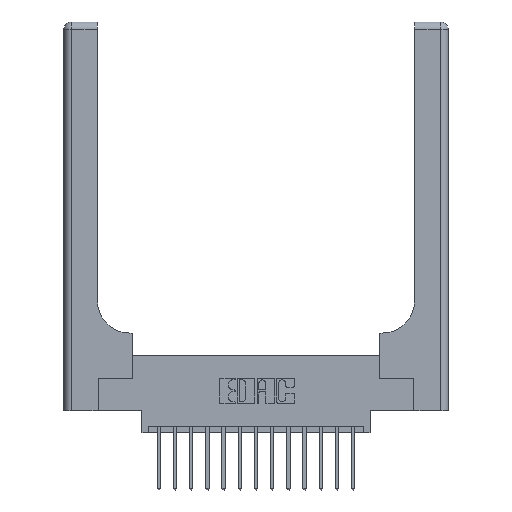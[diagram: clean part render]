
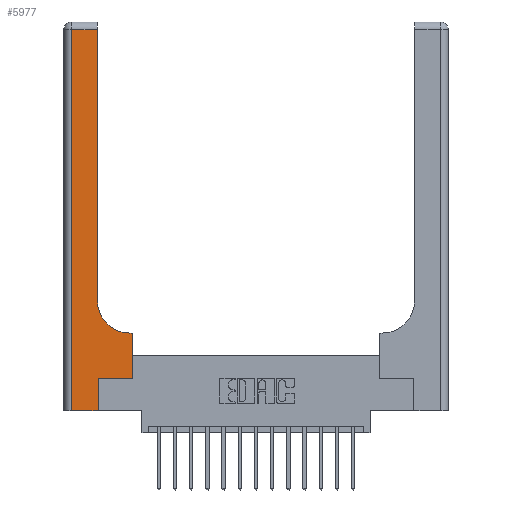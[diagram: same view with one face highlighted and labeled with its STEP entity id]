
A CAD part, top view. The second image highlights one B-rep face of the part: STEP entity #5977.
In plain terms, the highlighted planar face has unit normal (0, 0, 1).
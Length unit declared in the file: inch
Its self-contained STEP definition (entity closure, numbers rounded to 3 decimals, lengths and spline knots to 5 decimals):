
#105 = EDGE_CURVE ( 'NONE', #8761, #6554, #12553, .T. ) ;
#276 = EDGE_CURVE ( 'NONE', #6554, #7786, #18009, .T. ) ;
#674 = CARTESIAN_POINT ( 'NONE',  ( 0.06, 0., 0.37 ) ) ;
#1154 = ORIENTED_EDGE ( 'NONE', *, *, #7341, .T. ) ;
#1285 = EDGE_CURVE ( 'NONE', #2473, #6010, #10579, .T. ) ;
#1869 = AXIS2_PLACEMENT_3D ( 'NONE', #15434, #2851, #9680 ) ;
#2473 = VERTEX_POINT ( 'NONE', #8098 ) ;
#2480 = CARTESIAN_POINT ( 'NONE',  ( 0.26, 0.85, 0.37 ) ) ;
#2680 = DIRECTION ( 'NONE',  ( 0., 1., 0. ) ) ;
#2851 = DIRECTION ( 'NONE',  ( 0., 0., -1. ) ) ;
#3140 = DIRECTION ( 'NONE',  ( -1., 0., 0. ) ) ;
#3757 = VECTOR ( 'NONE', #4029, 39.37008 ) ;
#3887 = CARTESIAN_POINT ( 'NONE',  ( 0.265, 0., 0.37 ) ) ;
#3974 = LINE ( 'NONE', #3887, #14321 ) ;
#4029 = DIRECTION ( 'NONE',  ( 1., 0., 0. ) ) ;
#4353 = CARTESIAN_POINT ( 'NONE',  ( 0.26, 2.94, 0.37 ) ) ;
#4377 = LINE ( 'NONE', #7072, #3757 ) ;
#4520 = FACE_OUTER_BOUND ( 'NONE', #8047, .T. ) ;
#4982 = VECTOR ( 'NONE', #13230, 39.37008 ) ;
#5689 = EDGE_CURVE ( 'NONE', #13192, #17780, #13564, .T. ) ;
#5850 = CARTESIAN_POINT ( 'NONE',  ( 0.51, 0.6, 0.37 ) ) ;
#5942 = EDGE_CURVE ( 'NONE', #17780, #8761, #7209, .T. ) ;
#5977 = ADVANCED_FACE ( 'NONE', ( #4520 ), #10151, .F. ) ;
#6010 = VERTEX_POINT ( 'NONE', #674 ) ;
#6452 = CARTESIAN_POINT ( 'NONE',  ( 0.265, 0.25, 0.37 ) ) ;
#6554 = VERTEX_POINT ( 'NONE', #5850 ) ;
#7072 = CARTESIAN_POINT ( 'NONE',  ( 0., 0., 0.37 ) ) ;
#7209 = LINE ( 'NONE', #15556, #10176 ) ;
#7341 = EDGE_CURVE ( 'NONE', #9785, #13192, #3974, .T. ) ;
#7627 = CARTESIAN_POINT ( 'NONE',  ( 0., 2.94, 0.37 ) ) ;
#7652 = VECTOR ( 'NONE', #15150, 39.37008 ) ;
#7786 = VERTEX_POINT ( 'NONE', #2480 ) ;
#7792 = ORIENTED_EDGE ( 'NONE', *, *, #105, .T. ) ;
#7852 = EDGE_CURVE ( 'NONE', #7786, #9629, #8100, .T. ) ;
#7862 = DIRECTION ( 'NONE',  ( 1., 0., 0. ) ) ;
#7957 = CARTESIAN_POINT ( 'NONE',  ( 0.265, 0.25, 0.37 ) ) ;
#8010 = ORIENTED_EDGE ( 'NONE', *, *, #5942, .T. ) ;
#8047 = EDGE_LOOP ( 'NONE', ( #18118, #9099, #8105, #12429, #1154, #12051, #8010, #7792, #12926 ) ) ;
#8098 = CARTESIAN_POINT ( 'NONE',  ( 0.06, 2.94, 0.37 ) ) ;
#8100 = LINE ( 'NONE', #11119, #7652 ) ;
#8105 = ORIENTED_EDGE ( 'NONE', *, *, #1285, .T. ) ;
#8761 = VERTEX_POINT ( 'NONE', #17090 ) ;
#9042 = AXIS2_PLACEMENT_3D ( 'NONE', #15741, #15841, #3140 ) ;
#9099 = ORIENTED_EDGE ( 'NONE', *, *, #14943, .T. ) ;
#9197 = CARTESIAN_POINT ( 'NONE',  ( 0.528, 0.25, 0.37 ) ) ;
#9217 = DIRECTION ( 'NONE',  ( 0., -1., 0. ) ) ;
#9261 = EDGE_CURVE ( 'NONE', #6010, #9785, #4377, .T. ) ;
#9423 = DIRECTION ( 'NONE',  ( -1., 0., 0. ) ) ;
#9629 = VERTEX_POINT ( 'NONE', #4353 ) ;
#9680 = DIRECTION ( 'NONE',  ( 1., 0., 0. ) ) ;
#9785 = VERTEX_POINT ( 'NONE', #17226 ) ;
#10151 = PLANE ( 'NONE',  #9042 ) ;
#10176 = VECTOR ( 'NONE', #11524, 39.37008 ) ;
#10579 = LINE ( 'NONE', #11772, #15669 ) ;
#11119 = CARTESIAN_POINT ( 'NONE',  ( 0.26, 3., 0.37 ) ) ;
#11524 = DIRECTION ( 'NONE',  ( 0., 1., 0. ) ) ;
#11772 = CARTESIAN_POINT ( 'NONE',  ( 0.06, 3., 0.37 ) ) ;
#11940 = LINE ( 'NONE', #7627, #4982 ) ;
#12051 = ORIENTED_EDGE ( 'NONE', *, *, #5689, .T. ) ;
#12429 = ORIENTED_EDGE ( 'NONE', *, *, #9261, .T. ) ;
#12553 = LINE ( 'NONE', #17322, #16245 ) ;
#12926 = ORIENTED_EDGE ( 'NONE', *, *, #276, .T. ) ;
#13192 = VERTEX_POINT ( 'NONE', #6452 ) ;
#13230 = DIRECTION ( 'NONE',  ( -1., 0., 0. ) ) ;
#13564 = LINE ( 'NONE', #7957, #17055 ) ;
#14321 = VECTOR ( 'NONE', #2680, 39.37008 ) ;
#14943 = EDGE_CURVE ( 'NONE', #9629, #2473, #11940, .T. ) ;
#15150 = DIRECTION ( 'NONE',  ( 0., 1., 0. ) ) ;
#15434 = CARTESIAN_POINT ( 'NONE',  ( 0.51, 0.85, 0.37 ) ) ;
#15556 = CARTESIAN_POINT ( 'NONE',  ( 0.528, 0.25, 0.37 ) ) ;
#15669 = VECTOR ( 'NONE', #9217, 39.37008 ) ;
#15741 = CARTESIAN_POINT ( 'NONE',  ( 0., 3., 0.37 ) ) ;
#15841 = DIRECTION ( 'NONE',  ( 0., 0., -1. ) ) ;
#16245 = VECTOR ( 'NONE', #9423, 39.37008 ) ;
#17055 = VECTOR ( 'NONE', #7862, 39.37008 ) ;
#17090 = CARTESIAN_POINT ( 'NONE',  ( 0.528, 0.6, 0.37 ) ) ;
#17226 = CARTESIAN_POINT ( 'NONE',  ( 0.265, 0., 0.37 ) ) ;
#17322 = CARTESIAN_POINT ( 'NONE',  ( 0.26, 0.6, 0.37 ) ) ;
#17780 = VERTEX_POINT ( 'NONE', #9197 ) ;
#18009 = CIRCLE ( 'NONE', #1869, 0.25 ) ;
#18118 = ORIENTED_EDGE ( 'NONE', *, *, #7852, .T. ) ;
